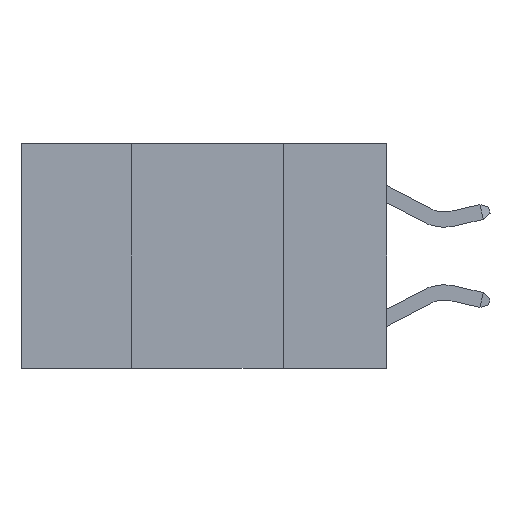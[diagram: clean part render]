
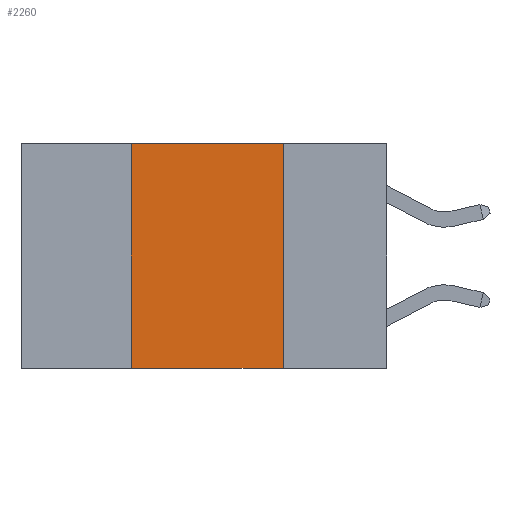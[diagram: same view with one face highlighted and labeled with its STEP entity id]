
A CAD part, left-side view. The second image highlights one B-rep face of the part: STEP entity #2260.
In plain terms, the highlighted planar face has unit normal (-1, 0, 0).
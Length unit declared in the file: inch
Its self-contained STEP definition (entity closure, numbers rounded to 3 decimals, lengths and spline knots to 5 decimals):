
#117 = EDGE_CURVE ( 'NONE', #22797, #4620, #643, .T. ) ;
#301 = ORIENTED_EDGE ( 'NONE', *, *, #10155, .T. ) ;
#643 = LINE ( 'NONE', #15161, #19247 ) ;
#815 = DIRECTION ( 'NONE',  ( 0., 0., -1. ) ) ;
#1433 = ORIENTED_EDGE ( 'NONE', *, *, #117, .F. ) ;
#1762 = CARTESIAN_POINT ( 'NONE',  ( 0., 0.17, 0. ) ) ;
#2260 = ADVANCED_FACE ( 'NONE', ( #17132 ), #21270, .F. ) ;
#2762 = CARTESIAN_POINT ( 'NONE',  ( 0., 0.17, -0.37 ) ) ;
#2805 = LINE ( 'NONE', #6581, #21396 ) ;
#3823 = VERTEX_POINT ( 'NONE', #7737 ) ;
#4620 = VERTEX_POINT ( 'NONE', #2762 ) ;
#4864 = ORIENTED_EDGE ( 'NONE', *, *, #10767, .F. ) ;
#4975 = CARTESIAN_POINT ( 'NONE',  ( 0., 0.6, 0. ) ) ;
#6581 = CARTESIAN_POINT ( 'NONE',  ( 0., 0.6, 0. ) ) ;
#6783 = VECTOR ( 'NONE', #12957, 39.37008 ) ;
#7522 = VERTEX_POINT ( 'NONE', #8606 ) ;
#7737 = CARTESIAN_POINT ( 'NONE',  ( 0., 0.42, -0.37 ) ) ;
#8372 = DIRECTION ( 'NONE',  ( 0., -1., 0. ) ) ;
#8606 = CARTESIAN_POINT ( 'NONE',  ( 0., 0.42, 0. ) ) ;
#8712 = EDGE_LOOP ( 'NONE', ( #1433, #4864, #18311, #301 ) ) ;
#10155 = EDGE_CURVE ( 'NONE', #3823, #4620, #20580, .T. ) ;
#10425 = DIRECTION ( 'NONE',  ( 1., 0., 0. ) ) ;
#10767 = EDGE_CURVE ( 'NONE', #7522, #22797, #2805, .T. ) ;
#12957 = DIRECTION ( 'NONE',  ( 0., 0., 1. ) ) ;
#15161 = CARTESIAN_POINT ( 'NONE',  ( 0., 0.17, 0. ) ) ;
#15747 = VECTOR ( 'NONE', #20858, 39.37008 ) ;
#17132 = FACE_OUTER_BOUND ( 'NONE', #8712, .T. ) ;
#18311 = ORIENTED_EDGE ( 'NONE', *, *, #22262, .F. ) ;
#19056 = CARTESIAN_POINT ( 'NONE',  ( 0., 0.6, -0.37 ) ) ;
#19220 = AXIS2_PLACEMENT_3D ( 'NONE', #4975, #10425, #23061 ) ;
#19247 = VECTOR ( 'NONE', #815, 39.37008 ) ;
#20580 = LINE ( 'NONE', #19056, #15747 ) ;
#20858 = DIRECTION ( 'NONE',  ( 0., -1., 0. ) ) ;
#21168 = LINE ( 'NONE', #21989, #6783 ) ;
#21270 = PLANE ( 'NONE',  #19220 ) ;
#21396 = VECTOR ( 'NONE', #8372, 39.37008 ) ;
#21989 = CARTESIAN_POINT ( 'NONE',  ( 0., 0.42, 0. ) ) ;
#22262 = EDGE_CURVE ( 'NONE', #3823, #7522, #21168, .T. ) ;
#22797 = VERTEX_POINT ( 'NONE', #1762 ) ;
#23061 = DIRECTION ( 'NONE',  ( 0., 0., -1. ) ) ;
